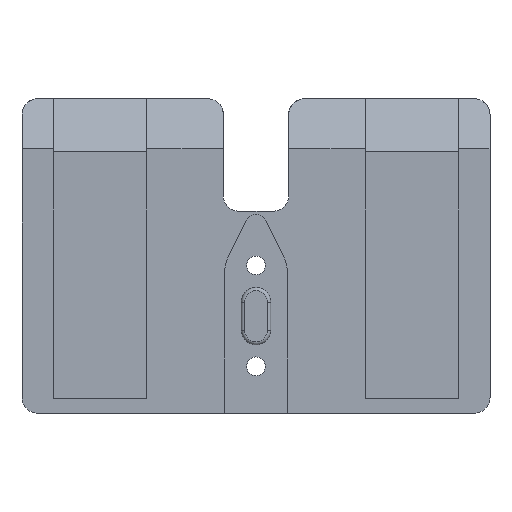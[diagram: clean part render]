
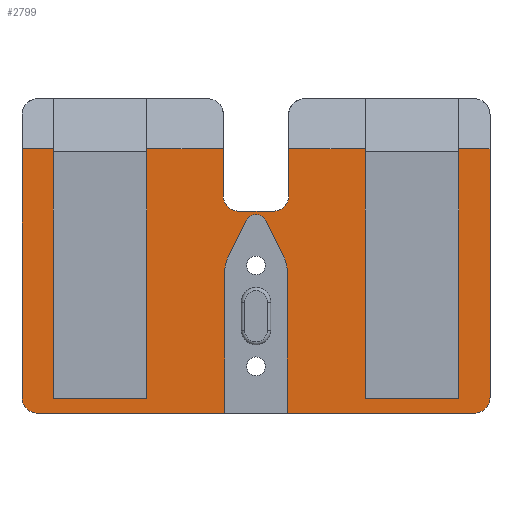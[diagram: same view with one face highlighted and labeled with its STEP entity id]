
A CAD part, front view. The second image highlights one B-rep face of the part: STEP entity #2799.
In plain terms, the highlighted planar face has unit normal (0, -1, 0).
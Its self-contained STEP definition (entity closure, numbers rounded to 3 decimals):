
#163=PLANE('',#3025);
#323=FACE_OUTER_BOUND('',#491,.T.);
#491=EDGE_LOOP('',(#2477,#2478,#2479,#2480,#2481,#2482,#2483,#2484,#2485,
#2486,#2487,#2488,#2489,#2490,#2491,#2492,#2493,#2494,#2495,#2496,#2497,
#2498,#2499,#2500,#2501,#2502,#2503,#2504));
#712=LINE('',#4663,#988);
#717=LINE('',#4674,#993);
#727=LINE('',#4699,#1003);
#736=LINE('',#4739,#1012);
#743=LINE('',#4764,#1019);
#745=LINE('',#4768,#1021);
#746=LINE('',#4770,#1022);
#747=LINE('',#4774,#1023);
#748=LINE('',#4776,#1024);
#749=LINE('',#4778,#1025);
#750=LINE('',#4780,#1026);
#751=LINE('',#4782,#1027);
#752=LINE('',#4784,#1028);
#753=LINE('',#4786,#1029);
#754=LINE('',#4789,#1030);
#755=LINE('',#4791,#1031);
#756=LINE('',#4793,#1032);
#757=LINE('',#4795,#1033);
#758=LINE('',#4796,#1034);
#759=LINE('',#4797,#1035);
#760=LINE('',#4799,#1036);
#988=VECTOR('',#3547,10.);
#993=VECTOR('',#3558,10.);
#1003=VECTOR('',#3580,10.);
#1012=VECTOR('',#3625,10.);
#1019=VECTOR('',#3648,10.);
#1021=VECTOR('',#3652,10.);
#1022=VECTOR('',#3653,10.);
#1023=VECTOR('',#3656,10.);
#1024=VECTOR('',#3657,10.);
#1025=VECTOR('',#3658,10.);
#1026=VECTOR('',#3659,10.);
#1027=VECTOR('',#3660,10.);
#1028=VECTOR('',#3661,10.);
#1029=VECTOR('',#3662,10.);
#1030=VECTOR('',#3665,10.);
#1031=VECTOR('',#3666,10.);
#1032=VECTOR('',#3667,10.);
#1033=VECTOR('',#3668,10.);
#1034=VECTOR('',#3669,10.);
#1035=VECTOR('',#3670,10.);
#1036=VECTOR('',#3671,10.);
#1135=CIRCLE('',#2991,2.5);
#1136=CIRCLE('',#3000,2.5);
#1146=CIRCLE('',#3015,5.);
#1151=CIRCLE('',#3023,5.);
#1152=CIRCLE('',#3026,2.5);
#1153=CIRCLE('',#3027,2.5);
#1154=CIRCLE('',#3028,1.75);
#1351=VERTEX_POINT('',#4660);
#1352=VERTEX_POINT('',#4662);
#1353=VERTEX_POINT('',#4666);
#1355=VERTEX_POINT('',#4672);
#1363=VERTEX_POINT('',#4696);
#1364=VERTEX_POINT('',#4698);
#1365=VERTEX_POINT('',#4702);
#1374=VERTEX_POINT('',#4729);
#1375=VERTEX_POINT('',#4731);
#1377=VERTEX_POINT('',#4737);
#1385=VERTEX_POINT('',#4757);
#1386=VERTEX_POINT('',#4759);
#1387=VERTEX_POINT('',#4763);
#1388=VERTEX_POINT('',#4767);
#1389=VERTEX_POINT('',#4769);
#1390=VERTEX_POINT('',#4771);
#1391=VERTEX_POINT('',#4773);
#1392=VERTEX_POINT('',#4775);
#1393=VERTEX_POINT('',#4777);
#1394=VERTEX_POINT('',#4779);
#1395=VERTEX_POINT('',#4781);
#1396=VERTEX_POINT('',#4783);
#1397=VERTEX_POINT('',#4785);
#1398=VERTEX_POINT('',#4788);
#1399=VERTEX_POINT('',#4790);
#1400=VERTEX_POINT('',#4792);
#1401=VERTEX_POINT('',#4794);
#1402=VERTEX_POINT('',#4798);
#1714=EDGE_CURVE('',#1351,#1352,#712,.T.);
#1717=EDGE_CURVE('',#1353,#1351,#1135,.T.);
#1720=EDGE_CURVE('',#1355,#1353,#717,.T.);
#1732=EDGE_CURVE('',#1364,#1363,#727,.T.);
#1735=EDGE_CURVE('',#1365,#1363,#1136,.T.);
#1748=EDGE_CURVE('',#1374,#1375,#1146,.F.);
#1752=EDGE_CURVE('',#1374,#1377,#736,.F.);
#1762=EDGE_CURVE('',#1385,#1386,#1151,.F.);
#1764=EDGE_CURVE('',#1387,#1386,#743,.F.);
#1766=EDGE_CURVE('',#1388,#1375,#745,.F.);
#1767=EDGE_CURVE('',#1377,#1389,#746,.T.);
#1768=EDGE_CURVE('',#1390,#1389,#1152,.T.);
#1769=EDGE_CURVE('',#1390,#1391,#747,.T.);
#1770=EDGE_CURVE('',#1392,#1391,#748,.T.);
#1771=EDGE_CURVE('',#1392,#1393,#749,.F.);
#1772=EDGE_CURVE('',#1393,#1394,#750,.F.);
#1773=EDGE_CURVE('',#1394,#1395,#751,.F.);
#1774=EDGE_CURVE('',#1396,#1395,#752,.T.);
#1775=EDGE_CURVE('',#1397,#1396,#753,.T.);
#1776=EDGE_CURVE('',#1352,#1397,#1153,.T.);
#1777=EDGE_CURVE('',#1398,#1355,#754,.T.);
#1778=EDGE_CURVE('',#1398,#1399,#755,.F.);
#1779=EDGE_CURVE('',#1399,#1400,#756,.F.);
#1780=EDGE_CURVE('',#1400,#1401,#757,.F.);
#1781=EDGE_CURVE('',#1364,#1401,#758,.T.);
#1782=EDGE_CURVE('',#1365,#1387,#759,.T.);
#1783=EDGE_CURVE('',#1385,#1402,#760,.F.);
#1784=EDGE_CURVE('',#1388,#1402,#1154,.F.);
#2477=ORIENTED_EDGE('',*,*,#1766,.T.);
#2478=ORIENTED_EDGE('',*,*,#1748,.F.);
#2479=ORIENTED_EDGE('',*,*,#1752,.T.);
#2480=ORIENTED_EDGE('',*,*,#1767,.T.);
#2481=ORIENTED_EDGE('',*,*,#1768,.F.);
#2482=ORIENTED_EDGE('',*,*,#1769,.T.);
#2483=ORIENTED_EDGE('',*,*,#1770,.F.);
#2484=ORIENTED_EDGE('',*,*,#1771,.T.);
#2485=ORIENTED_EDGE('',*,*,#1772,.T.);
#2486=ORIENTED_EDGE('',*,*,#1773,.T.);
#2487=ORIENTED_EDGE('',*,*,#1774,.F.);
#2488=ORIENTED_EDGE('',*,*,#1775,.F.);
#2489=ORIENTED_EDGE('',*,*,#1776,.F.);
#2490=ORIENTED_EDGE('',*,*,#1714,.F.);
#2491=ORIENTED_EDGE('',*,*,#1717,.F.);
#2492=ORIENTED_EDGE('',*,*,#1720,.F.);
#2493=ORIENTED_EDGE('',*,*,#1777,.F.);
#2494=ORIENTED_EDGE('',*,*,#1778,.T.);
#2495=ORIENTED_EDGE('',*,*,#1779,.T.);
#2496=ORIENTED_EDGE('',*,*,#1780,.T.);
#2497=ORIENTED_EDGE('',*,*,#1781,.F.);
#2498=ORIENTED_EDGE('',*,*,#1732,.T.);
#2499=ORIENTED_EDGE('',*,*,#1735,.F.);
#2500=ORIENTED_EDGE('',*,*,#1782,.T.);
#2501=ORIENTED_EDGE('',*,*,#1764,.T.);
#2502=ORIENTED_EDGE('',*,*,#1762,.F.);
#2503=ORIENTED_EDGE('',*,*,#1783,.T.);
#2504=ORIENTED_EDGE('',*,*,#1784,.F.);
#2799=ADVANCED_FACE('',(#323),#163,.F.);
#2991=AXIS2_PLACEMENT_3D('',#4668,#3552,#3553);
#3000=AXIS2_PLACEMENT_3D('',#4704,#3585,#3586);
#3015=AXIS2_PLACEMENT_3D('',#4732,#3618,#3619);
#3023=AXIS2_PLACEMENT_3D('',#4760,#3643,#3644);
#3025=AXIS2_PLACEMENT_3D('',#4766,#3650,#3651);
#3026=AXIS2_PLACEMENT_3D('',#4772,#3654,#3655);
#3027=AXIS2_PLACEMENT_3D('',#4787,#3663,#3664);
#3028=AXIS2_PLACEMENT_3D('',#4800,#3672,#3673);
#3547=DIRECTION('',(1.,0.,0.));
#3552=DIRECTION('center_axis',(0.,-1.,0.));
#3553=DIRECTION('ref_axis',(-0.707,0.,-0.707));
#3558=DIRECTION('',(0.,0.,-1.));
#3580=DIRECTION('',(0.,0.,-1.));
#3585=DIRECTION('center_axis',(0.,1.,0.));
#3586=DIRECTION('ref_axis',(-0.707,0.,-0.707));
#3618=DIRECTION('center_axis',(0.,1.,0.));
#3619=DIRECTION('ref_axis',(0.973,0.,0.23));
#3625=DIRECTION('',(0.,0.,1.));
#3643=DIRECTION('center_axis',(0.,1.,0.));
#3644=DIRECTION('ref_axis',(-0.973,0.,0.23));
#3648=DIRECTION('',(0.,0.,-1.));
#3650=DIRECTION('center_axis',(0.,1.,0.));
#3651=DIRECTION('ref_axis',(0.,0.,-1.));
#3652=DIRECTION('',(-0.447,0.,0.894));
#3653=DIRECTION('',(1.,0.,0.));
#3654=DIRECTION('center_axis',(0.,1.,0.));
#3655=DIRECTION('ref_axis',(0.707,0.,-0.707));
#3656=DIRECTION('',(0.,0.,1.));
#3657=DIRECTION('',(1.,0.,0.));
#3658=DIRECTION('',(0.,0.,1.));
#3659=DIRECTION('',(1.,0.,0.));
#3660=DIRECTION('',(0.,0.,-1.));
#3661=DIRECTION('',(1.,0.,0.));
#3662=DIRECTION('',(0.,0.,1.));
#3663=DIRECTION('center_axis',(0.,-1.,0.));
#3664=DIRECTION('ref_axis',(0.707,0.,-0.707));
#3665=DIRECTION('',(1.,0.,0.));
#3666=DIRECTION('',(0.,0.,1.));
#3667=DIRECTION('',(1.,0.,0.));
#3668=DIRECTION('',(0.,0.,-1.));
#3669=DIRECTION('',(1.,0.,0.));
#3670=DIRECTION('',(1.,0.,0.));
#3671=DIRECTION('',(-0.447,0.,-0.894));
#3672=DIRECTION('center_axis',(0.,1.,0.));
#3673=DIRECTION('ref_axis',(-0.894,0.,0.447));
#4660=CARTESIAN_POINT('',(42.25,30.,56.369));
#4662=CARTESIAN_POINT('',(47.75,30.,56.369));
#4663=CARTESIAN_POINT('',(44.25,30.,56.369));
#4666=CARTESIAN_POINT('',(39.75,30.,58.869));
#4668=CARTESIAN_POINT('Origin',(42.25,30.,58.869));
#4672=CARTESIAN_POINT('',(39.75,30.,66.369));
#4674=CARTESIAN_POINT('',(39.75,30.,59.369));
#4696=CARTESIAN_POINT('',(7.5,30.,26.5));
#4698=CARTESIAN_POINT('',(7.5,30.,66.369));
#4699=CARTESIAN_POINT('',(7.5,30.,47.369));
#4702=CARTESIAN_POINT('',(10.,30.,24.));
#4704=CARTESIAN_POINT('Origin',(10.,30.,26.5));
#4729=CARTESIAN_POINT('',(50.,30.,46.82));
#4731=CARTESIAN_POINT('',(49.472,30.,49.056));
#4732=CARTESIAN_POINT('Origin',(45.,30.,46.82));
#4737=CARTESIAN_POINT('',(50.,30.,24.));
#4739=CARTESIAN_POINT('',(50.,30.,41.685));
#4757=CARTESIAN_POINT('',(40.527,30.,49.056));
#4759=CARTESIAN_POINT('',(40.,30.,46.82));
#4760=CARTESIAN_POINT('Origin',(45.,30.,46.82));
#4763=CARTESIAN_POINT('',(40.,30.,24.));
#4764=CARTESIAN_POINT('',(40.,30.,41.685));
#4766=CARTESIAN_POINT('Origin',(44.25,30.,47.369));
#4767=CARTESIAN_POINT('',(46.565,30.,54.87));
#4768=CARTESIAN_POINT('',(48.926,30.,50.148));
#4769=CARTESIAN_POINT('',(80.,30.,24.));
#4770=CARTESIAN_POINT('',(44.25,30.,24.));
#4771=CARTESIAN_POINT('',(82.5,30.,26.5));
#4772=CARTESIAN_POINT('Origin',(80.,30.,26.5));
#4773=CARTESIAN_POINT('',(82.5,30.,66.369));
#4774=CARTESIAN_POINT('',(82.5,30.,47.369));
#4775=CARTESIAN_POINT('',(77.499,30.,66.369));
#4776=CARTESIAN_POINT('',(44.25,30.,66.369));
#4777=CARTESIAN_POINT('',(77.499,30.,26.369));
#4778=CARTESIAN_POINT('',(77.499,30.,48.119));
#4779=CARTESIAN_POINT('',(62.499,30.,26.369));
#4780=CARTESIAN_POINT('',(57.125,30.,26.369));
#4781=CARTESIAN_POINT('',(62.499,30.,66.369));
#4782=CARTESIAN_POINT('',(62.499,30.,48.119));
#4783=CARTESIAN_POINT('',(50.25,30.,66.369));
#4784=CARTESIAN_POINT('',(44.25,30.,66.369));
#4785=CARTESIAN_POINT('',(50.25,30.,58.869));
#4786=CARTESIAN_POINT('',(50.25,30.,59.369));
#4787=CARTESIAN_POINT('Origin',(47.75,30.,58.869));
#4788=CARTESIAN_POINT('',(27.5,30.,66.369));
#4789=CARTESIAN_POINT('',(44.25,30.,66.369));
#4790=CARTESIAN_POINT('',(27.5,30.,26.369));
#4791=CARTESIAN_POINT('',(27.5,30.,48.119));
#4792=CARTESIAN_POINT('',(12.5,30.,26.369));
#4793=CARTESIAN_POINT('',(32.125,30.,26.369));
#4794=CARTESIAN_POINT('',(12.5,30.,66.369));
#4795=CARTESIAN_POINT('',(12.5,30.,48.119));
#4796=CARTESIAN_POINT('',(44.25,30.,66.369));
#4797=CARTESIAN_POINT('',(44.25,30.,24.));
#4798=CARTESIAN_POINT('',(43.434,30.,54.87));
#4799=CARTESIAN_POINT('',(40.923,30.,49.848));
#4800=CARTESIAN_POINT('Origin',(45.,30.,54.087));
